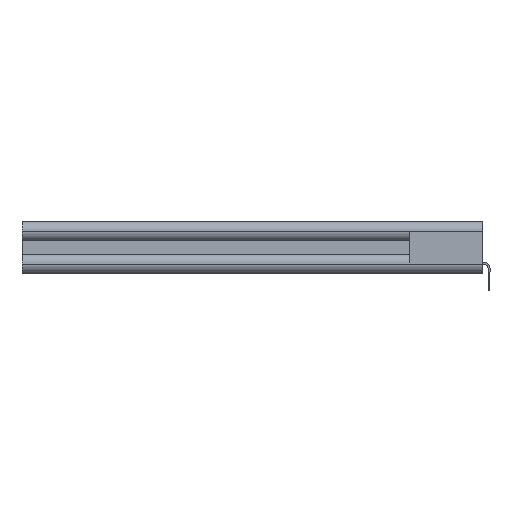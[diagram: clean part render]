
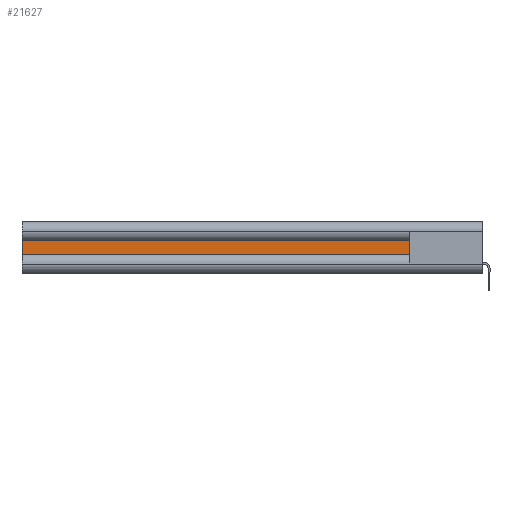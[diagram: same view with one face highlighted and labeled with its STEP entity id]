
A CAD part, left-side view. The second image highlights one B-rep face of the part: STEP entity #21627.
In plain terms, the highlighted planar face has unit normal (-1, 0, 0).
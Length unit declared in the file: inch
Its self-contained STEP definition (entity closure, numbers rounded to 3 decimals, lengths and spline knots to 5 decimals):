
#129 = DIRECTION ( 'NONE',  ( 0., 0., -1. ) ) ;
#273 = DIRECTION ( 'NONE',  ( 1., 0., 0. ) ) ;
#1444 = EDGE_CURVE ( 'NONE', #21393, #6012, #9295, .T. ) ;
#1671 = CARTESIAN_POINT ( 'NONE',  ( 0.044, 0.473, -0.0465 ) ) ;
#2694 = VERTEX_POINT ( 'NONE', #9715 ) ;
#4628 = LINE ( 'NONE', #23249, #23453 ) ;
#4736 = ORIENTED_EDGE ( 'NONE', *, *, #7275, .F. ) ;
#5573 = VERTEX_POINT ( 'NONE', #22150 ) ;
#6012 = VERTEX_POINT ( 'NONE', #19714 ) ;
#7275 = EDGE_CURVE ( 'NONE', #5573, #2694, #19463, .T. ) ;
#7400 = DIRECTION ( 'NONE',  ( 0., 0., -1. ) ) ;
#8133 = EDGE_CURVE ( 'NONE', #5573, #21393, #16080, .T. ) ;
#8447 = CARTESIAN_POINT ( 'NONE',  ( 0.044, 3., -0.0465 ) ) ;
#8718 = VECTOR ( 'NONE', #129, 39.37008 ) ;
#8949 = CARTESIAN_POINT ( 'NONE',  ( 0.044, 3., 0.0465 ) ) ;
#9295 = LINE ( 'NONE', #8447, #8718 ) ;
#9649 = CARTESIAN_POINT ( 'NONE',  ( 0.044, 0.37012, -0.0465 ) ) ;
#9715 = CARTESIAN_POINT ( 'NONE',  ( 0.044, 0.473, -0.0465 ) ) ;
#11221 = VECTOR ( 'NONE', #13319, 39.37008 ) ;
#11889 = EDGE_LOOP ( 'NONE', ( #17617, #15166, #18801, #4736 ) ) ;
#13319 = DIRECTION ( 'NONE',  ( 0., 1., 0. ) ) ;
#13346 = DIRECTION ( 'NONE',  ( 0., 0., -1. ) ) ;
#15166 = ORIENTED_EDGE ( 'NONE', *, *, #1444, .T. ) ;
#16080 = LINE ( 'NONE', #16946, #11221 ) ;
#16946 = CARTESIAN_POINT ( 'NONE',  ( 0.044, 0.37012, 0.0465 ) ) ;
#17617 = ORIENTED_EDGE ( 'NONE', *, *, #8133, .T. ) ;
#18801 = ORIENTED_EDGE ( 'NONE', *, *, #21365, .F. ) ;
#19463 = LINE ( 'NONE', #1671, #23638 ) ;
#19714 = CARTESIAN_POINT ( 'NONE',  ( 0.044, 3., -0.0465 ) ) ;
#20511 = PLANE ( 'NONE',  #23070 ) ;
#21365 = EDGE_CURVE ( 'NONE', #2694, #6012, #4628, .T. ) ;
#21393 = VERTEX_POINT ( 'NONE', #8949 ) ;
#21540 = DIRECTION ( 'NONE',  ( 0., 1., 0. ) ) ;
#21627 = ADVANCED_FACE ( 'NONE', ( #23718 ), #20511, .F. ) ;
#22150 = CARTESIAN_POINT ( 'NONE',  ( 0.044, 0.473, 0.0465 ) ) ;
#23070 = AXIS2_PLACEMENT_3D ( 'NONE', #9649, #273, #13346 ) ;
#23249 = CARTESIAN_POINT ( 'NONE',  ( 0.044, 0.37012, -0.0465 ) ) ;
#23453 = VECTOR ( 'NONE', #21540, 39.37008 ) ;
#23638 = VECTOR ( 'NONE', #7400, 39.37008 ) ;
#23718 = FACE_OUTER_BOUND ( 'NONE', #11889, .T. ) ;
